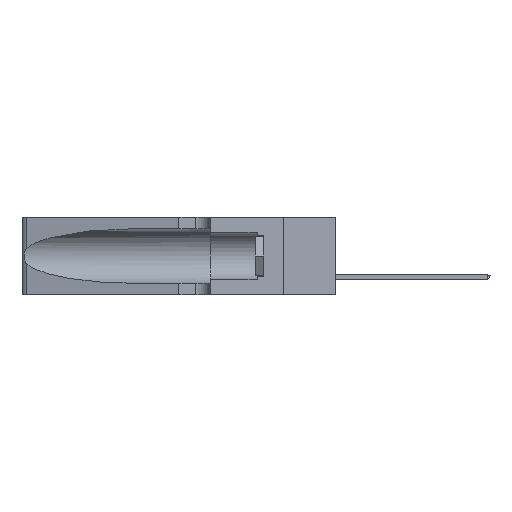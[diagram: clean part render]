
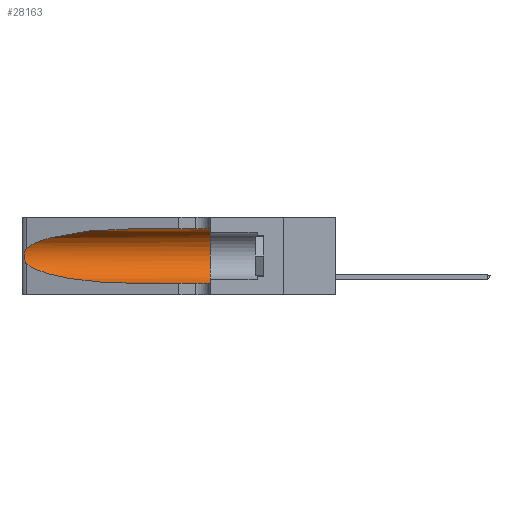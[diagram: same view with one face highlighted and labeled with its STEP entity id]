
A CAD part, left-side view. The second image highlights one B-rep face of the part: STEP entity #28163.
In plain terms, the highlighted cylindrical face has radius 3.308 mm (diameter 6.617 mm), a partial arc.
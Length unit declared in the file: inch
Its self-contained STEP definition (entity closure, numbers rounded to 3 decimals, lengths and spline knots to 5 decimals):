
#44 = EDGE_CURVE ( 'NONE', #23217, #5096, #3935, .T. ) ;
#197 = DIRECTION ( 'NONE',  ( 0., -1., 0. ) ) ;
#558 = CARTESIAN_POINT ( 'NONE',  ( 0.25854, 1.2359, 0.20912 ) ) ;
#1231 = FACE_OUTER_BOUND ( 'NONE', #31900, .T. ) ;
#1892 = CARTESIAN_POINT ( 'NONE',  ( 0.1305, 0.72297, 0.05475 ) ) ;
#2053 = CARTESIAN_POINT ( 'NONE',  ( 0.25555, 1.22993, 0.14849 ) ) ;
#3012 = CARTESIAN_POINT ( 'NONE',  ( 0.2373, 1.15595, 0.28018 ) ) ;
#3935 =( BOUNDED_CURVE ( )  B_SPLINE_CURVE ( 3, ( #24672, #30299, #17350, #14663 ),
 .UNSPECIFIED., .F., .T. ) 
 B_SPLINE_CURVE_WITH_KNOTS ( ( 4, 4 ),
 ( 3.44316, 4.71239 ),
 .UNSPECIFIED. ) 
 CURVE ( )  GEOMETRIC_REPRESENTATION_ITEM ( )  RATIONAL_B_SPLINE_CURVE ( ( 1., 0.87, 0.87, 1. ) ) 
 REPRESENTATION_ITEM ( '' )  );
#5078 = LINE ( 'NONE', #14620, #8722 ) ;
#5095 = DIRECTION ( 'NONE',  ( 0., 0., -1. ) ) ;
#5096 = VERTEX_POINT ( 'NONE', #1892 ) ;
#5956 = DIRECTION ( 'NONE',  ( 0., 1., 0. ) ) ;
#6376 = CARTESIAN_POINT ( 'NONE',  ( 0.1305, 0.72297, 0.31525 ) ) ;
#7345 = CYLINDRICAL_SURFACE ( 'NONE', #9343, 0.13025 ) ;
#7525 = EDGE_CURVE ( 'NONE', #25623, #23343, #20188, .T. ) ;
#7610 = ORIENTED_EDGE ( 'NONE', *, *, #25901, .T. ) ;
#8074 = CARTESIAN_POINT ( 'NONE',  ( 0.1305, 0.35, 0.31525 ) ) ;
#8722 = VECTOR ( 'NONE', #12204, 39.37008 ) ;
#9343 = AXIS2_PLACEMENT_3D ( 'NONE', #28359, #197, #5095 ) ;
#11620 = DIRECTION ( 'NONE',  ( 0., 0., 1. ) ) ;
#12123 = CARTESIAN_POINT ( 'NONE',  ( 0.25487, 1.22718, 0.14631 ) ) ;
#12190 = ORIENTED_EDGE ( 'NONE', *, *, #44, .T. ) ;
#12204 = DIRECTION ( 'NONE',  ( 0., -1., 0. ) ) ;
#12891 = CARTESIAN_POINT ( 'NONE',  ( 0.1305, 1.61858, 0.31525 ) ) ;
#13225 = CARTESIAN_POINT ( 'NONE',  ( 0.25487, 1.22718, 0.22369 ) ) ;
#13342 = EDGE_CURVE ( 'NONE', #18610, #23217, #27165, .T. ) ;
#13850 = CARTESIAN_POINT ( 'NONE',  ( 0.26018, 1.23835, 0.19895 ) ) ;
#14165 = ORIENTED_EDGE ( 'NONE', *, *, #21018, .T. ) ;
#14620 = CARTESIAN_POINT ( 'NONE',  ( 0.1305, 1.61858, 0.05475 ) ) ;
#14663 = CARTESIAN_POINT ( 'NONE',  ( 0.1305, 0.72297, 0.05475 ) ) ;
#14903 = CARTESIAN_POINT ( 'NONE',  ( 0.25639, 1.23186, 0.15144 ) ) ;
#15999 = CARTESIAN_POINT ( 'NONE',  ( 0.25487, 1.22718, 0.22369 ) ) ;
#16115 = VECTOR ( 'NONE', #18955, 39.37008 ) ;
#16564 = CARTESIAN_POINT ( 'NONE',  ( 0.26017, 1.23833, 0.17102 ) ) ;
#16791 = CARTESIAN_POINT ( 'NONE',  ( 0.26075, 1.23896, 0.178 ) ) ;
#17056 = AXIS2_PLACEMENT_3D ( 'NONE', #29415, #5956, #11620 ) ;
#17350 = CARTESIAN_POINT ( 'NONE',  ( 0.18966, 0.96281, 0.05475 ) ) ;
#18610 = VERTEX_POINT ( 'NONE', #19734 ) ;
#18955 = DIRECTION ( 'NONE',  ( 0., -1., 0. ) ) ;
#19734 = CARTESIAN_POINT ( 'NONE',  ( 0.25487, 1.22718, 0.22369 ) ) ;
#20188 = LINE ( 'NONE', #12891, #16115 ) ;
#21018 = EDGE_CURVE ( 'NONE', #25623, #18610, #25544, .T. ) ;
#21092 = EDGE_CURVE ( 'NONE', #23343, #30209, #23781, .T. ) ;
#21339 = CARTESIAN_POINT ( 'NONE',  ( 0.18966, 0.96281, 0.31525 ) ) ;
#22547 = ORIENTED_EDGE ( 'NONE', *, *, #21092, .F. ) ;
#22724 = CARTESIAN_POINT ( 'NONE',  ( 0.1305, 0.35, 0.05475 ) ) ;
#22764 = CARTESIAN_POINT ( 'NONE',  ( 0.25487, 1.22718, 0.14631 ) ) ;
#23217 = VERTEX_POINT ( 'NONE', #12123 ) ;
#23343 = VERTEX_POINT ( 'NONE', #8074 ) ;
#23781 = CIRCLE ( 'NONE', #17056, 0.13025 ) ;
#24672 = CARTESIAN_POINT ( 'NONE',  ( 0.25487, 1.22718, 0.14631 ) ) ;
#25317 = ORIENTED_EDGE ( 'NONE', *, *, #7525, .F. ) ;
#25544 =( BOUNDED_CURVE ( )  B_SPLINE_CURVE ( 3, ( #26224, #21339, #3012, #13225 ),
 .UNSPECIFIED., .F., .T. ) 
 B_SPLINE_CURVE_WITH_KNOTS ( ( 4, 4 ),
 ( 1.5708, 2.84003 ),
 .UNSPECIFIED. ) 
 CURVE ( )  GEOMETRIC_REPRESENTATION_ITEM ( )  RATIONAL_B_SPLINE_CURVE ( ( 1., 0.87, 0.87, 1. ) ) 
 REPRESENTATION_ITEM ( '' )  );
#25623 = VERTEX_POINT ( 'NONE', #6376 ) ;
#25752 = ORIENTED_EDGE ( 'NONE', *, *, #13342, .T. ) ;
#25901 = EDGE_CURVE ( 'NONE', #5096, #30209, #5078, .T. ) ;
#26224 = CARTESIAN_POINT ( 'NONE',  ( 0.1305, 0.72297, 0.31525 ) ) ;
#27165 = B_SPLINE_CURVE_WITH_KNOTS ( 'NONE', 3,
 ( #15999, #31631, #29362, #29250, #558, #13850, #29952, #16791, #16564, #32547, #27659, #14903, #2053, #22764 ),
 .UNSPECIFIED., .F., .F.,
 ( 4, 2, 2, 2, 2, 2, 4 ),
 ( 0., 0.00027, 0.00053, 0.00107, 0.0016, 0.00187, 0.00214 ),
 .UNSPECIFIED. ) ;
#27659 = CARTESIAN_POINT ( 'NONE',  ( 0.25789, 1.23486, 0.15765 ) ) ;
#28163 = ADVANCED_FACE ( 'NONE', ( #1231 ), #7345, .F. ) ;
#28359 = CARTESIAN_POINT ( 'NONE',  ( 0.1305, 1.61858, 0.185 ) ) ;
#29250 = CARTESIAN_POINT ( 'NONE',  ( 0.25787, 1.23484, 0.2124 ) ) ;
#29362 = CARTESIAN_POINT ( 'NONE',  ( 0.25639, 1.23184, 0.21858 ) ) ;
#29415 = CARTESIAN_POINT ( 'NONE',  ( 0.1305, 0.35, 0.185 ) ) ;
#29952 = CARTESIAN_POINT ( 'NONE',  ( 0.26075, 1.23896, 0.19203 ) ) ;
#30209 = VERTEX_POINT ( 'NONE', #22724 ) ;
#30299 = CARTESIAN_POINT ( 'NONE',  ( 0.2373, 1.15595, 0.08982 ) ) ;
#31631 = CARTESIAN_POINT ( 'NONE',  ( 0.25555, 1.22994, 0.2215 ) ) ;
#31900 = EDGE_LOOP ( 'NONE', ( #14165, #25752, #12190, #7610, #22547, #25317 ) ) ;
#32547 = CARTESIAN_POINT ( 'NONE',  ( 0.25856, 1.23593, 0.16098 ) ) ;
